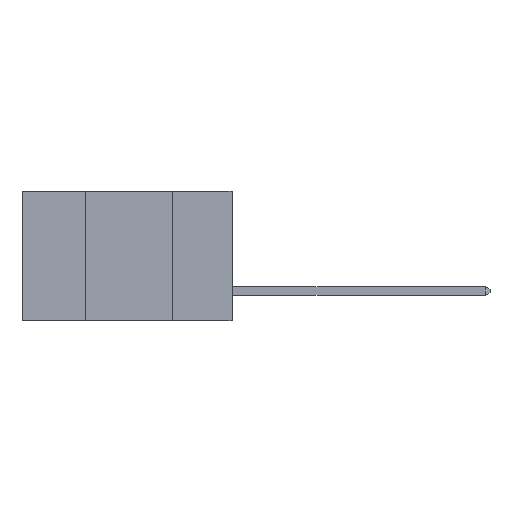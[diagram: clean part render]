
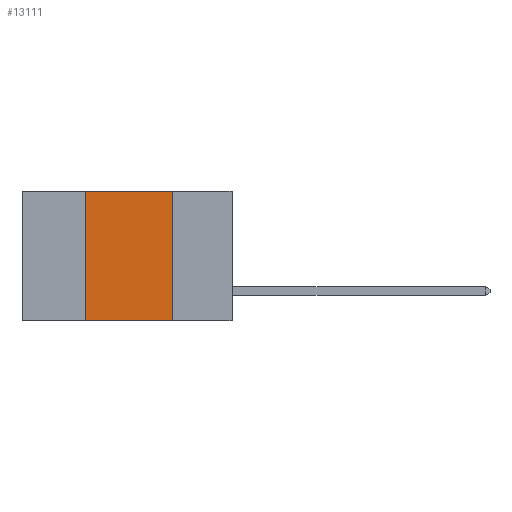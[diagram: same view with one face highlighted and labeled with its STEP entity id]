
A CAD part, left-side view. The second image highlights one B-rep face of the part: STEP entity #13111.
In plain terms, the highlighted planar face has unit normal (-1, 0, 0).
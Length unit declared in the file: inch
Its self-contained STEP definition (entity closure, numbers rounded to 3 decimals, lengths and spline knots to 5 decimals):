
#122 = LINE ( 'NONE', #13571, #9422 ) ;
#338 = VERTEX_POINT ( 'NONE', #9504 ) ;
#479 = FACE_OUTER_BOUND ( 'NONE', #5050, .T. ) ;
#991 = ORIENTED_EDGE ( 'NONE', *, *, #10637, .T. ) ;
#2175 = LINE ( 'NONE', #12209, #11396 ) ;
#2181 = DIRECTION ( 'NONE',  ( 0., -1., 0. ) ) ;
#2481 = PLANE ( 'NONE',  #11785 ) ;
#3058 = VECTOR ( 'NONE', #9917, 39.37008 ) ;
#3684 = ORIENTED_EDGE ( 'NONE', *, *, #13545, .F. ) ;
#4197 = CARTESIAN_POINT ( 'NONE',  ( 0., 0.42, 0. ) ) ;
#5050 = EDGE_LOOP ( 'NONE', ( #3684, #9761, #10111, #991 ) ) ;
#5687 = VECTOR ( 'NONE', #5863, 39.37008 ) ;
#5863 = DIRECTION ( 'NONE',  ( 0., 0., -1. ) ) ;
#5885 = CARTESIAN_POINT ( 'NONE',  ( 0., 0.42, -0.37 ) ) ;
#6610 = LINE ( 'NONE', #4197, #3058 ) ;
#6707 = DIRECTION ( 'NONE',  ( 0., -1., 0. ) ) ;
#7101 = CARTESIAN_POINT ( 'NONE',  ( 0., 0.17, -0.37 ) ) ;
#8433 = DIRECTION ( 'NONE',  ( 0., 0., -1. ) ) ;
#9422 = VECTOR ( 'NONE', #2181, 39.37008 ) ;
#9504 = CARTESIAN_POINT ( 'NONE',  ( 0., 0.17, 0. ) ) ;
#9761 = ORIENTED_EDGE ( 'NONE', *, *, #13400, .F. ) ;
#9917 = DIRECTION ( 'NONE',  ( 0., 0., 1. ) ) ;
#10111 = ORIENTED_EDGE ( 'NONE', *, *, #12113, .F. ) ;
#10279 = CARTESIAN_POINT ( 'NONE',  ( 0., 0.17, 0. ) ) ;
#10637 = EDGE_CURVE ( 'NONE', #14659, #10693, #122, .T. ) ;
#10693 = VERTEX_POINT ( 'NONE', #7101 ) ;
#11391 = CARTESIAN_POINT ( 'NONE',  ( 0., 0.42, 0. ) ) ;
#11396 = VECTOR ( 'NONE', #6707, 39.37008 ) ;
#11785 = AXIS2_PLACEMENT_3D ( 'NONE', #12783, #14900, #8433 ) ;
#12113 = EDGE_CURVE ( 'NONE', #14659, #14654, #6610, .T. ) ;
#12209 = CARTESIAN_POINT ( 'NONE',  ( 0., 0.6, 0. ) ) ;
#12783 = CARTESIAN_POINT ( 'NONE',  ( 0., 0.6, 0. ) ) ;
#13111 = ADVANCED_FACE ( 'NONE', ( #479 ), #2481, .F. ) ;
#13400 = EDGE_CURVE ( 'NONE', #14654, #338, #2175, .T. ) ;
#13545 = EDGE_CURVE ( 'NONE', #338, #10693, #14428, .T. ) ;
#13571 = CARTESIAN_POINT ( 'NONE',  ( 0., 0.6, -0.37 ) ) ;
#14428 = LINE ( 'NONE', #10279, #5687 ) ;
#14654 = VERTEX_POINT ( 'NONE', #11391 ) ;
#14659 = VERTEX_POINT ( 'NONE', #5885 ) ;
#14900 = DIRECTION ( 'NONE',  ( 1., 0., 0. ) ) ;
